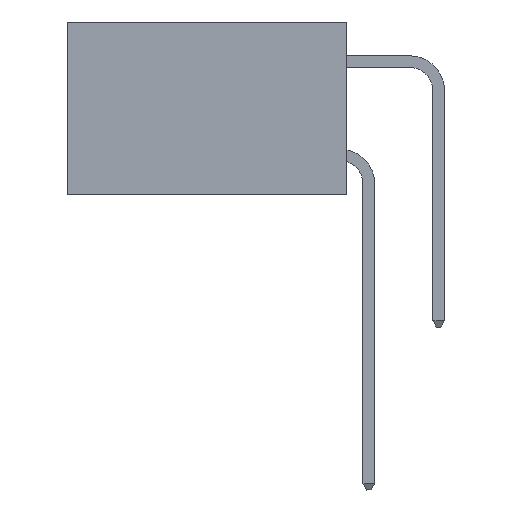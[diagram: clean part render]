
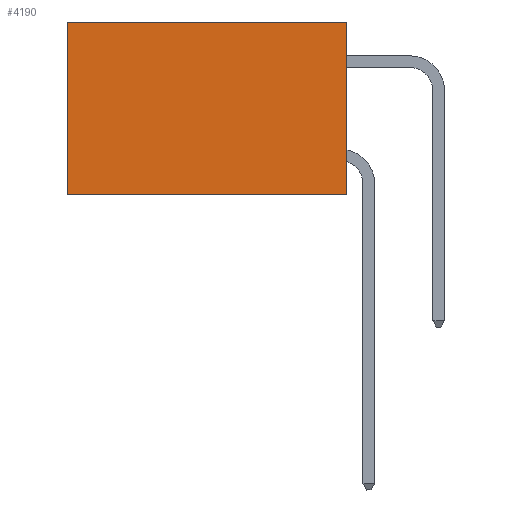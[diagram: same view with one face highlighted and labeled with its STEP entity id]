
A CAD part, left-side view. The second image highlights one B-rep face of the part: STEP entity #4190.
In plain terms, the highlighted planar face has unit normal (-1, 0, 0).
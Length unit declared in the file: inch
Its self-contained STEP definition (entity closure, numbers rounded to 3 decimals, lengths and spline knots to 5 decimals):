
#172 = VERTEX_POINT ( 'NONE', #2520 ) ;
#694 = VERTEX_POINT ( 'NONE', #12905 ) ;
#863 = LINE ( 'NONE', #3345, #8920 ) ;
#875 = EDGE_CURVE ( 'NONE', #172, #694, #7099, .T. ) ;
#1632 = ORIENTED_EDGE ( 'NONE', *, *, #6647, .T. ) ;
#1762 = CARTESIAN_POINT ( 'NONE',  ( 0.2875, 0., -0.37 ) ) ;
#1860 = VECTOR ( 'NONE', #10216, 39.37008 ) ;
#2301 = DIRECTION ( 'NONE',  ( 0., 0., -1. ) ) ;
#2520 = CARTESIAN_POINT ( 'NONE',  ( 0.2875, 0.6, 0. ) ) ;
#3345 = CARTESIAN_POINT ( 'NONE',  ( 0.2875, 0., 0. ) ) ;
#3649 = EDGE_CURVE ( 'NONE', #13485, #694, #7131, .T. ) ;
#4081 = VERTEX_POINT ( 'NONE', #12676 ) ;
#4190 = ADVANCED_FACE ( 'NONE', ( #5464 ), #5949, .F. ) ;
#4897 = VECTOR ( 'NONE', #9766, 39.37008 ) ;
#5464 = FACE_OUTER_BOUND ( 'NONE', #11065, .T. ) ;
#5795 = AXIS2_PLACEMENT_3D ( 'NONE', #12410, #12561, #12531 ) ;
#5949 = PLANE ( 'NONE',  #5795 ) ;
#6647 = EDGE_CURVE ( 'NONE', #4081, #172, #13047, .T. ) ;
#6807 = ORIENTED_EDGE ( 'NONE', *, *, #3649, .F. ) ;
#7099 = LINE ( 'NONE', #10587, #12111 ) ;
#7131 = LINE ( 'NONE', #1762, #1860 ) ;
#8713 = CARTESIAN_POINT ( 'NONE',  ( 0.2875, 0., 0. ) ) ;
#8920 = VECTOR ( 'NONE', #2301, 39.37008 ) ;
#9290 = EDGE_CURVE ( 'NONE', #4081, #13485, #863, .T. ) ;
#9766 = DIRECTION ( 'NONE',  ( 0., 1., 0. ) ) ;
#10216 = DIRECTION ( 'NONE',  ( 0., 1., 0. ) ) ;
#10587 = CARTESIAN_POINT ( 'NONE',  ( 0.2875, 0.6, 0. ) ) ;
#10764 = CARTESIAN_POINT ( 'NONE',  ( 0.2875, 0., -0.37 ) ) ;
#11065 = EDGE_LOOP ( 'NONE', ( #13057, #6807, #12700, #1632 ) ) ;
#12111 = VECTOR ( 'NONE', #12326, 39.37008 ) ;
#12326 = DIRECTION ( 'NONE',  ( 0., 0., -1. ) ) ;
#12410 = CARTESIAN_POINT ( 'NONE',  ( 0.2875, 0., 0. ) ) ;
#12531 = DIRECTION ( 'NONE',  ( 0., 0., -1. ) ) ;
#12561 = DIRECTION ( 'NONE',  ( 1., 0., 0. ) ) ;
#12676 = CARTESIAN_POINT ( 'NONE',  ( 0.2875, 0., 0. ) ) ;
#12700 = ORIENTED_EDGE ( 'NONE', *, *, #9290, .F. ) ;
#12905 = CARTESIAN_POINT ( 'NONE',  ( 0.2875, 0.6, -0.37 ) ) ;
#13047 = LINE ( 'NONE', #8713, #4897 ) ;
#13057 = ORIENTED_EDGE ( 'NONE', *, *, #875, .T. ) ;
#13485 = VERTEX_POINT ( 'NONE', #10764 ) ;
